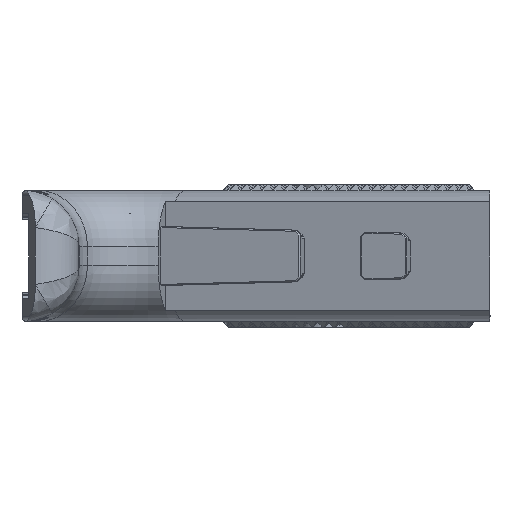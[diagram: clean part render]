
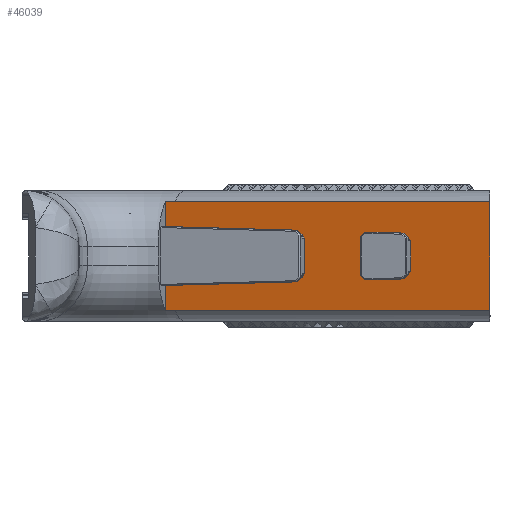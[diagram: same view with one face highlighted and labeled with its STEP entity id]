
A CAD part, left-side view. The second image highlights one B-rep face of the part: STEP entity #46039.
In plain terms, the highlighted planar face has unit normal (-0.951, 0.309, 0).
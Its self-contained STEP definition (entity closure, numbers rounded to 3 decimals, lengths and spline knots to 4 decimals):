
#88=FACE_BOUND('',#19694,.T.);
#2636=PLANE('',#49007);
#7569=LINE('',#88176,#13121);
#7670=LINE('',#88429,#13222);
#7688=LINE('',#88467,#13240);
#7696=LINE('',#88484,#13248);
#7701=LINE('',#88493,#13253);
#7703=LINE('',#88496,#13255);
#7705=LINE('',#88501,#13257);
#7707=LINE('',#88505,#13259);
#7709=LINE('',#88508,#13261);
#7711=LINE('',#88512,#13263);
#7712=LINE('',#88514,#13264);
#7718=LINE('',#88527,#13270);
#7720=LINE('',#88531,#13272);
#7721=LINE('',#88534,#13273);
#7723=LINE('',#88538,#13275);
#7724=LINE('',#88547,#13276);
#7725=LINE('',#88549,#13277);
#7726=LINE('',#88559,#13278);
#7727=LINE('',#88560,#13279);
#13121=VECTOR('',#59270,0.3937);
#13222=VECTOR('',#59457,0.3937);
#13240=VECTOR('',#59493,0.3937);
#13248=VECTOR('',#59507,0.3937);
#13253=VECTOR('',#59516,0.3937);
#13255=VECTOR('',#59520,0.3937);
#13257=VECTOR('',#59524,0.3937);
#13259=VECTOR('',#59528,0.3937);
#13261=VECTOR('',#59532,0.3937);
#13263=VECTOR('',#59536,0.3937);
#13264=VECTOR('',#59539,0.3937);
#13270=VECTOR('',#59555,0.3937);
#13272=VECTOR('',#59559,0.3937);
#13273=VECTOR('',#59562,0.3937);
#13275=VECTOR('',#59566,0.3937);
#13276=VECTOR('',#59567,0.3937);
#13277=VECTOR('',#59568,0.3937);
#13278=VECTOR('',#59569,0.3937);
#13279=VECTOR('',#59570,0.3937);
#16700=FACE_OUTER_BOUND('',#19693,.T.);
#19693=EDGE_LOOP('',(#41115,#41116,#41117,#41118,#41119,#41120,#41121,#41122,
#41123,#41124,#41125,#41126));
#19694=EDGE_LOOP('',(#41127,#41128,#41129,#41130,#41131,#41132,#41133,#41134,
#41135));
#20478=B_SPLINE_CURVE_WITH_KNOTS('',3,(#88540,#88541,#88542,#88543,#88544,
#88545,#88546),.UNSPECIFIED.,.F.,.F.,(4,3,4),(0.,0.1181,0.2155),
 .UNSPECIFIED.);
#20479=B_SPLINE_CURVE_WITH_KNOTS('',3,(#88551,#88552,#88553,#88554,#88555,
#88556,#88557),.UNSPECIFIED.,.F.,.F.,(4,3,4),(-0.2155,-0.1181,
0.),.UNSPECIFIED.);
#23422=VERTEX_POINT('',#88173);
#23423=VERTEX_POINT('',#88175);
#23500=VERTEX_POINT('',#88426);
#23501=VERTEX_POINT('',#88428);
#23511=VERTEX_POINT('',#88464);
#23512=VERTEX_POINT('',#88466);
#23517=VERTEX_POINT('',#88481);
#23518=VERTEX_POINT('',#88483);
#23520=VERTEX_POINT('',#88492);
#23521=VERTEX_POINT('',#88498);
#23522=VERTEX_POINT('',#88500);
#23523=VERTEX_POINT('',#88504);
#23524=VERTEX_POINT('',#88510);
#23526=VERTEX_POINT('',#88525);
#23527=VERTEX_POINT('',#88529);
#23528=VERTEX_POINT('',#88533);
#23529=VERTEX_POINT('',#88537);
#23530=VERTEX_POINT('',#88539);
#23531=VERTEX_POINT('',#88548);
#23532=VERTEX_POINT('',#88550);
#23533=VERTEX_POINT('',#88558);
#29354=EDGE_CURVE('',#23422,#23423,#7569,.T.);
#29466=EDGE_CURVE('',#23501,#23500,#7670,.T.);
#29484=EDGE_CURVE('',#23511,#23512,#7688,.T.);
#29492=EDGE_CURVE('',#23517,#23518,#7696,.F.);
#29497=EDGE_CURVE('',#23501,#23520,#7701,.F.);
#29499=EDGE_CURVE('',#23517,#23520,#7703,.T.);
#29501=EDGE_CURVE('',#23521,#23522,#7705,.F.);
#29503=EDGE_CURVE('',#23523,#23522,#7707,.T.);
#29505=EDGE_CURVE('',#23521,#23518,#7709,.T.);
#29507=EDGE_CURVE('',#23524,#23500,#7711,.F.);
#29508=EDGE_CURVE('',#23523,#23524,#7712,.F.);
#29514=EDGE_CURVE('',#23526,#23511,#7718,.F.);
#29516=EDGE_CURVE('',#23526,#23527,#7720,.T.);
#29517=EDGE_CURVE('',#23512,#23528,#7721,.F.);
#29519=EDGE_CURVE('',#23529,#23527,#7723,.T.);
#29520=EDGE_CURVE('',#23530,#23529,#20478,.T.);
#29521=EDGE_CURVE('',#23423,#23530,#7724,.T.);
#29522=EDGE_CURVE('',#23531,#23422,#7725,.T.);
#29523=EDGE_CURVE('',#23532,#23531,#20479,.T.);
#29524=EDGE_CURVE('',#23533,#23532,#7726,.T.);
#29525=EDGE_CURVE('',#23533,#23528,#7727,.T.);
#41115=ORIENTED_EDGE('',*,*,#29516,.T.);
#41116=ORIENTED_EDGE('',*,*,#29519,.F.);
#41117=ORIENTED_EDGE('',*,*,#29520,.F.);
#41118=ORIENTED_EDGE('',*,*,#29521,.F.);
#41119=ORIENTED_EDGE('',*,*,#29354,.F.);
#41120=ORIENTED_EDGE('',*,*,#29522,.F.);
#41121=ORIENTED_EDGE('',*,*,#29523,.F.);
#41122=ORIENTED_EDGE('',*,*,#29524,.F.);
#41123=ORIENTED_EDGE('',*,*,#29525,.T.);
#41124=ORIENTED_EDGE('',*,*,#29517,.F.);
#41125=ORIENTED_EDGE('',*,*,#29484,.F.);
#41126=ORIENTED_EDGE('',*,*,#29514,.F.);
#41127=ORIENTED_EDGE('',*,*,#29466,.T.);
#41128=ORIENTED_EDGE('',*,*,#29507,.F.);
#41129=ORIENTED_EDGE('',*,*,#29508,.F.);
#41130=ORIENTED_EDGE('',*,*,#29503,.T.);
#41131=ORIENTED_EDGE('',*,*,#29501,.F.);
#41132=ORIENTED_EDGE('',*,*,#29505,.T.);
#41133=ORIENTED_EDGE('',*,*,#29492,.F.);
#41134=ORIENTED_EDGE('',*,*,#29499,.T.);
#41135=ORIENTED_EDGE('',*,*,#29497,.F.);
#46039=ADVANCED_FACE('',(#16700,#88),#2636,.T.);
#49007=AXIS2_PLACEMENT_3D('',#88536,#59564,#59565);
#59270=DIRECTION('',(0.,0.,-1.));
#59457=DIRECTION('',(0.,0.,1.));
#59493=DIRECTION('',(0.,0.,1.));
#59507=DIRECTION('',(0.216,0.664,-0.716));
#59516=DIRECTION('',(0.221,0.681,0.698));
#59520=DIRECTION('',(0.309,0.951,-0.026));
#59524=DIRECTION('',(-0.216,-0.664,-0.716));
#59528=DIRECTION('',(-0.309,-0.951,-0.026));
#59532=DIRECTION('',(0.,0.,-1.));
#59536=DIRECTION('',(-0.12,-0.37,0.921));
#59539=DIRECTION('',(-0.221,-0.681,0.698));
#59555=DIRECTION('',(0.216,0.664,-0.716));
#59559=DIRECTION('',(0.309,0.951,-0.026));
#59562=DIRECTION('',(-0.216,-0.664,-0.716));
#59564=DIRECTION('center_axis',(-0.951,0.309,0.));
#59565=DIRECTION('ref_axis',(0.,0.,
1.));
#59566=DIRECTION('',(0.,0.,1.));
#59567=DIRECTION('',(0.309,0.951,0.));
#59568=DIRECTION('',(-0.309,-0.951,0.));
#59569=DIRECTION('',(0.,0.,1.));
#59570=DIRECTION('',(-0.309,-0.951,-0.026));
#88173=CARTESIAN_POINT('',(-3.2516,-1.9775,-0.2929));
#88175=CARTESIAN_POINT('',(-3.2516,-1.9775,-1.2425));
#88176=CARTESIAN_POINT('',(-3.2516,-1.9775,-0.3839));
#88426=CARTESIAN_POINT('',(-2.8962,-0.8838,-0.6352));
#88428=CARTESIAN_POINT('',(-2.8962,-0.8838,-0.9101));
#88429=CARTESIAN_POINT('',(-2.8962,-0.8838,-0.7677));
#88464=CARTESIAN_POINT('',(-2.7262,-0.3607,-0.9245));
#88466=CARTESIAN_POINT('',(-2.7262,-0.3607,-0.6109));
#88467=CARTESIAN_POINT('',(-2.7262,-0.3607,-0.9154));
#88481=CARTESIAN_POINT('',(-3.0247,-1.2792,-0.909));
#88483=CARTESIAN_POINT('',(-3.0277,-1.2886,-0.8989));
#88484=CARTESIAN_POINT('',(-2.9908,-1.1749,-1.0217));
#88492=CARTESIAN_POINT('',(-2.8992,-0.8932,-0.9197));
#88493=CARTESIAN_POINT('',(-2.8709,-0.806,-0.8303));
#88496=CARTESIAN_POINT('',(-3.0469,-1.3476,-0.9072));
#88498=CARTESIAN_POINT('',(-3.0277,-1.2886,-0.6365));
#88500=CARTESIAN_POINT('',(-3.0247,-1.2792,-0.6264));
#88501=CARTESIAN_POINT('',(-2.9908,-1.1749,-0.5138));
#88504=CARTESIAN_POINT('',(-2.8992,-0.8932,-0.6158));
#88505=CARTESIAN_POINT('',(-3.0469,-1.3476,-0.6283));
#88508=CARTESIAN_POINT('',(-3.0277,-1.2886,-0.899));
#88510=CARTESIAN_POINT('',(-2.8984,-0.8905,-0.6185));
#88512=CARTESIAN_POINT('',(-2.885,-0.8493,-0.7213));
#88514=CARTESIAN_POINT('',(-2.8709,-0.806,-0.7051));
#88525=CARTESIAN_POINT('',(-2.7232,-0.3514,-0.9346));
#88527=CARTESIAN_POINT('',(-2.7647,-0.479,-0.7968));
#88529=CARTESIAN_POINT('',(-2.3324,0.8513,-0.9677));
#88531=CARTESIAN_POINT('',(-3.0469,-1.3476,-0.9072));
#88533=CARTESIAN_POINT('',(-2.7232,-0.3514,-0.6008));
#88534=CARTESIAN_POINT('',(-2.7647,-0.479,-0.7386));
#88536=CARTESIAN_POINT('Origin',(-2.8375,-0.7031,-0.7677));
#88537=CARTESIAN_POINT('',(-2.3324,0.8513,-1.2459));
#88538=CARTESIAN_POINT('',(-2.3324,0.8513,-1.0302));
#88539=CARTESIAN_POINT('',(-2.3592,0.7689,-1.2425));
#88540=CARTESIAN_POINT('Ctrl Pts',(-2.3592,0.7689,
-1.2425));
#88541=CARTESIAN_POINT('Ctrl Pts',(-2.3544,0.7836,
-1.2425));
#88542=CARTESIAN_POINT('Ctrl Pts',(-2.3495,0.7986,
-1.2428));
#88543=CARTESIAN_POINT('Ctrl Pts',(-2.3446,0.8138,
-1.2435));
#88544=CARTESIAN_POINT('Ctrl Pts',(-2.3405,0.8264,
-1.2441));
#88545=CARTESIAN_POINT('Ctrl Pts',(-2.3365,0.8388,
-1.2449));
#88546=CARTESIAN_POINT('Ctrl Pts',(-2.3324,0.8513,-1.2459));
#88547=CARTESIAN_POINT('',(-2.1969,1.2684,-1.2425));
#88548=CARTESIAN_POINT('',(-2.3592,0.7689,-0.2929));
#88549=CARTESIAN_POINT('',(-2.6906,-0.2509,-0.2929));
#88550=CARTESIAN_POINT('',(-2.3324,0.8513,-0.2895));
#88551=CARTESIAN_POINT('Ctrl Pts',(-2.3324,0.8513,-0.2895));
#88552=CARTESIAN_POINT('Ctrl Pts',(-2.3365,0.8388,
-0.2905));
#88553=CARTESIAN_POINT('Ctrl Pts',(-2.3405,0.8264,
-0.2913));
#88554=CARTESIAN_POINT('Ctrl Pts',(-2.3446,0.8138,
-0.2919));
#88555=CARTESIAN_POINT('Ctrl Pts',(-2.3495,0.7986,
-0.2926));
#88556=CARTESIAN_POINT('Ctrl Pts',(-2.3544,0.7836,
-0.2929));
#88557=CARTESIAN_POINT('Ctrl Pts',(-2.3592,0.7689,
-0.2929));
#88558=CARTESIAN_POINT('',(-2.3324,0.8513,-0.5677));
#88559=CARTESIAN_POINT('',(-2.3324,0.8513,-0.7677));
#88560=CARTESIAN_POINT('',(-3.0469,-1.3476,-0.6283));
